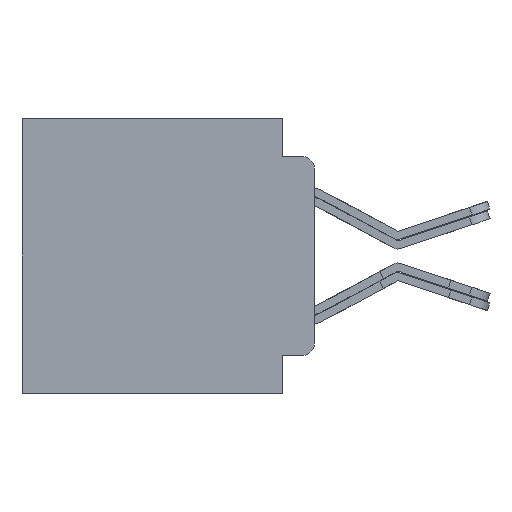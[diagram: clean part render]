
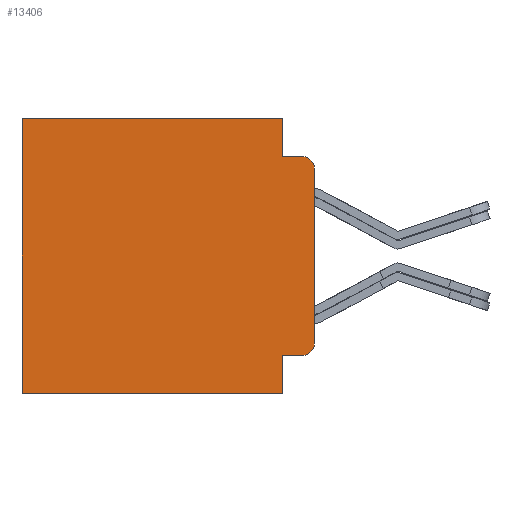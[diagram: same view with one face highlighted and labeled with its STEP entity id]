
A CAD part, left-side view. The second image highlights one B-rep face of the part: STEP entity #13406.
In plain terms, the highlighted planar face has unit normal (-1, 0, 0).
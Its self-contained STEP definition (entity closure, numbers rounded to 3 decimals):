
#805 = ORIENTED_EDGE ( 'NONE', *, *, #25626, .T. ) ;
#899 = ORIENTED_EDGE ( 'NONE', *, *, #9647, .F. ) ;
#1293 = LINE ( 'NONE', #19465, #27437 ) ;
#1471 = CARTESIAN_POINT ( 'NONE',  ( -67.462, 0., -3.467 ) ) ;
#1642 = CARTESIAN_POINT ( 'NONE',  ( -67.462, 0.508, 3.467 ) ) ;
#1737 = DIRECTION ( 'NONE',  ( -1., 0., 0. ) ) ;
#1820 = DIRECTION ( 'NONE',  ( 0., -1., 0. ) ) ;
#2208 = EDGE_CURVE ( 'NONE', #13373, #15379, #17181, .T. ) ;
#2308 = VERTEX_POINT ( 'NONE', #16997 ) ;
#2504 = LINE ( 'NONE', #22926, #8083 ) ;
#4125 = DIRECTION ( 'NONE',  ( 0., 0., -1. ) ) ;
#4305 = ORIENTED_EDGE ( 'NONE', *, *, #24197, .F. ) ;
#4846 = LINE ( 'NONE', #13204, #15986 ) ;
#5561 = CARTESIAN_POINT ( 'NONE',  ( -67.462, 1.295, 3.975 ) ) ;
#5651 = CARTESIAN_POINT ( 'NONE',  ( -67.462, 11.684, 5.486 ) ) ;
#6213 = AXIS2_PLACEMENT_3D ( 'NONE', #20106, #9150, #20402 ) ;
#7636 = DIRECTION ( 'NONE',  ( 0., -1., 0. ) ) ;
#7796 = ORIENTED_EDGE ( 'NONE', *, *, #25599, .T. ) ;
#7815 = CARTESIAN_POINT ( 'NONE',  ( -67.462, 1.295, 5.486 ) ) ;
#8083 = VECTOR ( 'NONE', #20976, 1000. ) ;
#8273 = CARTESIAN_POINT ( 'NONE',  ( -67.462, 1.295, -3.975 ) ) ;
#8756 = LINE ( 'NONE', #15140, #22281 ) ;
#8981 = LINE ( 'NONE', #14165, #22170 ) ;
#9150 = DIRECTION ( 'NONE',  ( -1., 0., 0. ) ) ;
#9455 = VERTEX_POINT ( 'NONE', #1471 ) ;
#9514 = CARTESIAN_POINT ( 'NONE',  ( -67.462, 0., -5.486 ) ) ;
#9647 = EDGE_CURVE ( 'NONE', #28678, #21913, #8756, .T. ) ;
#9698 = VERTEX_POINT ( 'NONE', #8273 ) ;
#10817 = EDGE_CURVE ( 'NONE', #16780, #9455, #4846, .T. ) ;
#11207 = ORIENTED_EDGE ( 'NONE', *, *, #10817, .F. ) ;
#12069 = AXIS2_PLACEMENT_3D ( 'NONE', #1642, #1737, #28044 ) ;
#12814 = DIRECTION ( 'NONE',  ( 0., 0., -1. ) ) ;
#13204 = CARTESIAN_POINT ( 'NONE',  ( -67.462, 0., -5.486 ) ) ;
#13373 = VERTEX_POINT ( 'NONE', #5651 ) ;
#13406 = ADVANCED_FACE ( 'NONE', ( #20116 ), #14558, .F. ) ;
#13643 = ORIENTED_EDGE ( 'NONE', *, *, #22591, .T. ) ;
#13855 = EDGE_CURVE ( 'NONE', #15018, #13373, #8981, .T. ) ;
#14165 = CARTESIAN_POINT ( 'NONE',  ( -67.462, 0., 5.486 ) ) ;
#14558 = PLANE ( 'NONE',  #14568 ) ;
#14568 = AXIS2_PLACEMENT_3D ( 'NONE', #16620, #16531, #16909 ) ;
#15018 = VERTEX_POINT ( 'NONE', #7815 ) ;
#15140 = CARTESIAN_POINT ( 'NONE',  ( -67.462, 1.295, 3.975 ) ) ;
#15379 = VERTEX_POINT ( 'NONE', #17676 ) ;
#15986 = VECTOR ( 'NONE', #12814, 1000. ) ;
#16297 = DIRECTION ( 'NONE',  ( 0., 1., 0. ) ) ;
#16517 = CIRCLE ( 'NONE', #12069, 0.508 ) ;
#16531 = DIRECTION ( 'NONE',  ( 1., 0., 0. ) ) ;
#16564 = DIRECTION ( 'NONE',  ( 0., 0., -1. ) ) ;
#16620 = CARTESIAN_POINT ( 'NONE',  ( -67.462, 0., -5.486 ) ) ;
#16780 = VERTEX_POINT ( 'NONE', #22019 ) ;
#16909 = DIRECTION ( 'NONE',  ( 0., 0., -1. ) ) ;
#16997 = CARTESIAN_POINT ( 'NONE',  ( -67.462, 0.508, -3.975 ) ) ;
#17181 = LINE ( 'NONE', #25118, #25901 ) ;
#17676 = CARTESIAN_POINT ( 'NONE',  ( -67.462, 11.684, -5.486 ) ) ;
#18889 = VERTEX_POINT ( 'NONE', #27585 ) ;
#19465 = CARTESIAN_POINT ( 'NONE',  ( -67.462, 1.295, 0. ) ) ;
#20106 = CARTESIAN_POINT ( 'NONE',  ( -67.462, 0.508, -3.467 ) ) ;
#20116 = FACE_OUTER_BOUND ( 'NONE', #25847, .T. ) ;
#20247 = EDGE_CURVE ( 'NONE', #18889, #15379, #25551, .T. ) ;
#20402 = DIRECTION ( 'NONE',  ( 0., 0., -1. ) ) ;
#20671 = DIRECTION ( 'NONE',  ( 0., 1., 0. ) ) ;
#20804 = ORIENTED_EDGE ( 'NONE', *, *, #20247, .F. ) ;
#20976 = DIRECTION ( 'NONE',  ( 0., 0., -1. ) ) ;
#21017 = VECTOR ( 'NONE', #16297, 1000. ) ;
#21289 = CARTESIAN_POINT ( 'NONE',  ( -67.462, 1.295, -3.975 ) ) ;
#21628 = EDGE_CURVE ( 'NONE', #9698, #18889, #2504, .T. ) ;
#21855 = ORIENTED_EDGE ( 'NONE', *, *, #13855, .T. ) ;
#21913 = VERTEX_POINT ( 'NONE', #22562 ) ;
#22019 = CARTESIAN_POINT ( 'NONE',  ( -67.462, 0., 3.467 ) ) ;
#22170 = VECTOR ( 'NONE', #20671, 1000. ) ;
#22281 = VECTOR ( 'NONE', #1820, 1000. ) ;
#22562 = CARTESIAN_POINT ( 'NONE',  ( -67.462, 0.508, 3.975 ) ) ;
#22591 = EDGE_CURVE ( 'NONE', #2308, #9455, #23631, .T. ) ;
#22926 = CARTESIAN_POINT ( 'NONE',  ( -67.462, 1.295, 0. ) ) ;
#23263 = ORIENTED_EDGE ( 'NONE', *, *, #21628, .F. ) ;
#23631 = CIRCLE ( 'NONE', #6213, 0.508 ) ;
#24197 = EDGE_CURVE ( 'NONE', #15018, #28678, #1293, .T. ) ;
#25118 = CARTESIAN_POINT ( 'NONE',  ( -67.462, 11.684, -5.486 ) ) ;
#25551 = LINE ( 'NONE', #9514, #21017 ) ;
#25599 = EDGE_CURVE ( 'NONE', #9698, #2308, #28366, .T. ) ;
#25626 = EDGE_CURVE ( 'NONE', #16780, #21913, #16517, .T. ) ;
#25847 = EDGE_LOOP ( 'NONE', ( #7796, #13643, #11207, #805, #899, #4305, #21855, #27538, #20804, #23263 ) ) ;
#25901 = VECTOR ( 'NONE', #16564, 1000. ) ;
#27437 = VECTOR ( 'NONE', #4125, 1000. ) ;
#27538 = ORIENTED_EDGE ( 'NONE', *, *, #2208, .T. ) ;
#27585 = CARTESIAN_POINT ( 'NONE',  ( -67.462, 1.295, -5.486 ) ) ;
#27683 = VECTOR ( 'NONE', #7636, 1000. ) ;
#28044 = DIRECTION ( 'NONE',  ( 0., 0., -1. ) ) ;
#28366 = LINE ( 'NONE', #21289, #27683 ) ;
#28678 = VERTEX_POINT ( 'NONE', #5561 ) ;
